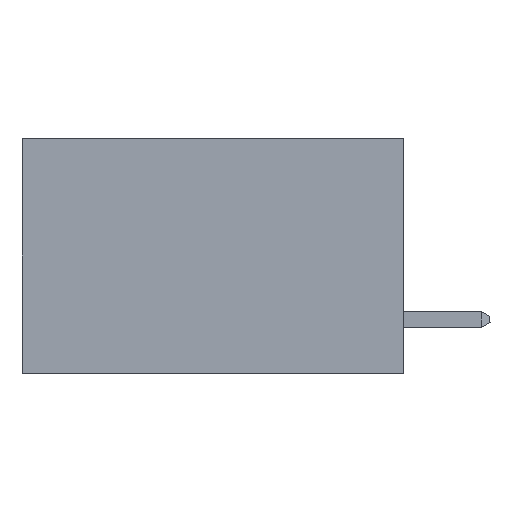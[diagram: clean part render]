
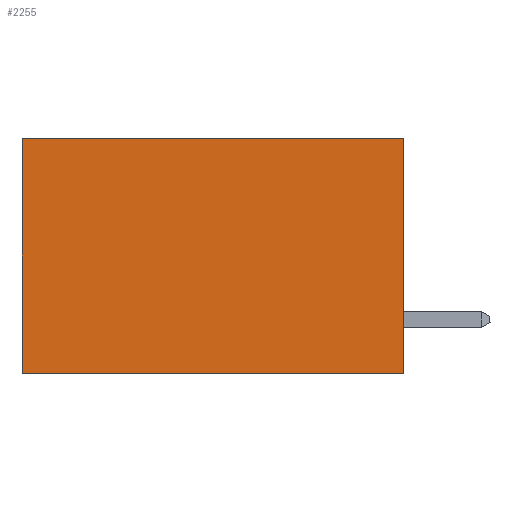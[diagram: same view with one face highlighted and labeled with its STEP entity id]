
A CAD part, left-side view. The second image highlights one B-rep face of the part: STEP entity #2255.
In plain terms, the highlighted planar face has unit normal (-1, 0, 0).
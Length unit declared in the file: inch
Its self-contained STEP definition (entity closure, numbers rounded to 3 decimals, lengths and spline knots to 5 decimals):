
#471 = CARTESIAN_POINT ( 'NONE',  ( 0.2875, 0., 0. ) ) ;
#578 = VERTEX_POINT ( 'NONE', #8558 ) ;
#1044 = VERTEX_POINT ( 'NONE', #8316 ) ;
#2255 = ADVANCED_FACE ( 'NONE', ( #7837 ), #7381, .F. ) ;
#2350 = DIRECTION ( 'NONE',  ( 0., 0., -1. ) ) ;
#2773 = ORIENTED_EDGE ( 'NONE', *, *, #3905, .T. ) ;
#3905 = EDGE_CURVE ( 'NONE', #9375, #578, #8334, .T. ) ;
#3962 = DIRECTION ( 'NONE',  ( 1., 0., 0. ) ) ;
#3998 = VECTOR ( 'NONE', #6348, 39.37008 ) ;
#4114 = DIRECTION ( 'NONE',  ( 0., 1., 0. ) ) ;
#4968 = ORIENTED_EDGE ( 'NONE', *, *, #5182, .F. ) ;
#5182 = EDGE_CURVE ( 'NONE', #1044, #6999, #8969, .T. ) ;
#5529 = VECTOR ( 'NONE', #10314, 39.37008 ) ;
#6348 = DIRECTION ( 'NONE',  ( 0., 1., 0. ) ) ;
#6999 = VERTEX_POINT ( 'NONE', #17028 ) ;
#7262 = EDGE_CURVE ( 'NONE', #578, #6999, #8891, .T. ) ;
#7381 = PLANE ( 'NONE',  #8822 ) ;
#7837 = FACE_OUTER_BOUND ( 'NONE', #14074, .T. ) ;
#8316 = CARTESIAN_POINT ( 'NONE',  ( 0.2875, 0., -0.37 ) ) ;
#8334 = LINE ( 'NONE', #13145, #3998 ) ;
#8558 = CARTESIAN_POINT ( 'NONE',  ( 0.2875, 0.6, 0. ) ) ;
#8822 = AXIS2_PLACEMENT_3D ( 'NONE', #471, #3962, #2350 ) ;
#8891 = LINE ( 'NONE', #10427, #9313 ) ;
#8969 = LINE ( 'NONE', #17508, #12970 ) ;
#9313 = VECTOR ( 'NONE', #9480, 39.37008 ) ;
#9375 = VERTEX_POINT ( 'NONE', #16052 ) ;
#9471 = ORIENTED_EDGE ( 'NONE', *, *, #7262, .T. ) ;
#9480 = DIRECTION ( 'NONE',  ( 0., 0., -1. ) ) ;
#10314 = DIRECTION ( 'NONE',  ( 0., 0., -1. ) ) ;
#10422 = CARTESIAN_POINT ( 'NONE',  ( 0.2875, 0., 0. ) ) ;
#10427 = CARTESIAN_POINT ( 'NONE',  ( 0.2875, 0.6, 0. ) ) ;
#10458 = EDGE_CURVE ( 'NONE', #9375, #1044, #15783, .T. ) ;
#12970 = VECTOR ( 'NONE', #4114, 39.37008 ) ;
#13145 = CARTESIAN_POINT ( 'NONE',  ( 0.2875, 0., 0. ) ) ;
#14074 = EDGE_LOOP ( 'NONE', ( #9471, #4968, #15178, #2773 ) ) ;
#15178 = ORIENTED_EDGE ( 'NONE', *, *, #10458, .F. ) ;
#15783 = LINE ( 'NONE', #10422, #5529 ) ;
#16052 = CARTESIAN_POINT ( 'NONE',  ( 0.2875, 0., 0. ) ) ;
#17028 = CARTESIAN_POINT ( 'NONE',  ( 0.2875, 0.6, -0.37 ) ) ;
#17508 = CARTESIAN_POINT ( 'NONE',  ( 0.2875, 0., -0.37 ) ) ;
